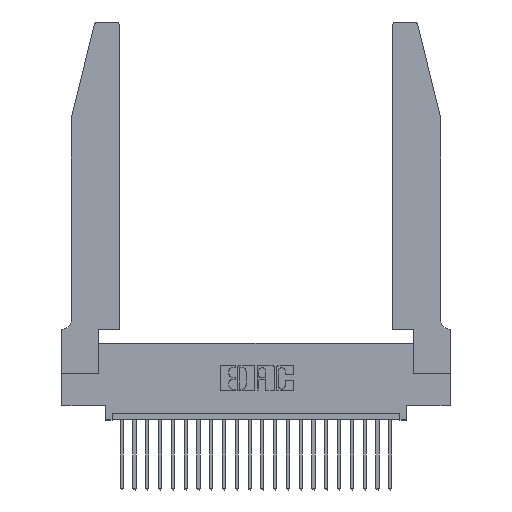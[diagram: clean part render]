
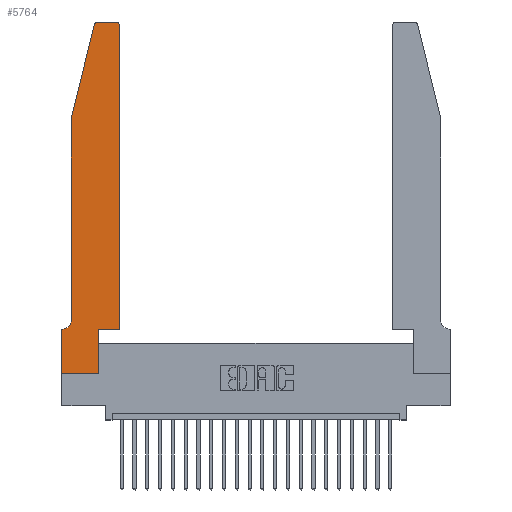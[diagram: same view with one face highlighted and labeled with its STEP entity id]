
A CAD part, top view. The second image highlights one B-rep face of the part: STEP entity #5764.
In plain terms, the highlighted planar face has unit normal (0, 0, 1).
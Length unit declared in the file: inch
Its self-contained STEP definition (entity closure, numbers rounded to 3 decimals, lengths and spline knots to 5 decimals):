
#12 = DIRECTION ( 'NONE',  ( 0., 0., 1. ) ) ;
#119 = EDGE_CURVE ( 'NONE', #18789, #23798, #5246, .T. ) ;
#302 = VECTOR ( 'NONE', #23434, 39.37008 ) ;
#432 = EDGE_CURVE ( 'NONE', #23798, #5064, #21632, .T. ) ;
#566 = VERTEX_POINT ( 'NONE', #6598 ) ;
#702 = EDGE_CURVE ( 'NONE', #5064, #22696, #14632, .T. ) ;
#795 = ORIENTED_EDGE ( 'NONE', *, *, #19122, .T. ) ;
#945 = VERTEX_POINT ( 'NONE', #11610 ) ;
#1464 = CARTESIAN_POINT ( 'NONE',  ( 0.0755, 2., 0.37 ) ) ;
#1549 = DIRECTION ( 'NONE',  ( 1., 0., 0. ) ) ;
#2223 = DIRECTION ( 'NONE',  ( 1., 0., 0. ) ) ;
#2553 = CARTESIAN_POINT ( 'NONE',  ( 0.0755, 0.42, 0.37 ) ) ;
#2623 = ORIENTED_EDGE ( 'NONE', *, *, #15102, .T. ) ;
#2695 = VECTOR ( 'NONE', #16484, 39.37008 ) ;
#2698 = ORIENTED_EDGE ( 'NONE', *, *, #7828, .T. ) ;
#2810 = DIRECTION ( 'NONE',  ( 1., 0., 0. ) ) ;
#2921 = VECTOR ( 'NONE', #13179, 39.37008 ) ;
#3017 = CARTESIAN_POINT ( 'NONE',  ( 0.0755, 2., 0.37 ) ) ;
#3178 = VECTOR ( 'NONE', #5280, 39.37008 ) ;
#3492 = ORIENTED_EDGE ( 'NONE', *, *, #9373, .T. ) ;
#4136 = DIRECTION ( 'NONE',  ( 0., 1., 0. ) ) ;
#4333 = CIRCLE ( 'NONE', #5457, 0.03 ) ;
#4637 = VERTEX_POINT ( 'NONE', #20187 ) ;
#4794 = CARTESIAN_POINT ( 'NONE',  ( 0., 0.35, 0.37 ) ) ;
#4965 = CARTESIAN_POINT ( 'NONE',  ( 0., 0., 0.37 ) ) ;
#5064 = VERTEX_POINT ( 'NONE', #14235 ) ;
#5246 = LINE ( 'NONE', #9996, #302 ) ;
#5280 = DIRECTION ( 'NONE',  ( -0.239, -0.971, 0. ) ) ;
#5457 = AXIS2_PLACEMENT_3D ( 'NONE', #12424, #21608, #2810 ) ;
#5468 = CARTESIAN_POINT ( 'NONE',  ( 0.2605, 2.75, 0.37 ) ) ;
#5632 = EDGE_CURVE ( 'NONE', #21778, #21929, #9237, .T. ) ;
#5662 = VECTOR ( 'NONE', #16864, 39.37008 ) ;
#5764 = ADVANCED_FACE ( 'NONE', ( #15664 ), #17740, .T. ) ;
#6284 = CARTESIAN_POINT ( 'NONE',  ( 0.2865, 0.35, 0.37 ) ) ;
#6301 = AXIS2_PLACEMENT_3D ( 'NONE', #13717, #21052, #11763 ) ;
#6598 = CARTESIAN_POINT ( 'NONE',  ( 0.4505, 2.72, 0.37 ) ) ;
#6871 = EDGE_LOOP ( 'NONE', ( #10457, #3492, #2623, #7031, #16558, #19944, #7434, #2698, #12664, #17879, #9995, #795 ) ) ;
#7031 = ORIENTED_EDGE ( 'NONE', *, *, #119, .T. ) ;
#7434 = ORIENTED_EDGE ( 'NONE', *, *, #8720, .T. ) ;
#7692 = LINE ( 'NONE', #4965, #2695 ) ;
#7712 = DIRECTION ( 'NONE',  ( 0., 1., 0. ) ) ;
#7788 = CARTESIAN_POINT ( 'NONE',  ( 0.4505, 0.35, 0.37 ) ) ;
#7828 = EDGE_CURVE ( 'NONE', #945, #21778, #7692, .T. ) ;
#7903 = LINE ( 'NONE', #1464, #3178 ) ;
#8044 = VECTOR ( 'NONE', #4136, 39.37008 ) ;
#8320 = CARTESIAN_POINT ( 'NONE',  ( 0.25487, 2.72718, 0.37 ) ) ;
#8557 = AXIS2_PLACEMENT_3D ( 'NONE', #10317, #10395, #1549 ) ;
#8720 = EDGE_CURVE ( 'NONE', #22696, #945, #19917, .T. ) ;
#8729 = DIRECTION ( 'NONE',  ( -1., 0., 0. ) ) ;
#9237 = LINE ( 'NONE', #6284, #8044 ) ;
#9296 = CARTESIAN_POINT ( 'NONE',  ( 0.2865, 0., 0.37 ) ) ;
#9363 = LINE ( 'NONE', #7788, #18984 ) ;
#9373 = EDGE_CURVE ( 'NONE', #21474, #12568, #4333, .T. ) ;
#9563 = CARTESIAN_POINT ( 'NONE',  ( 0., 0., 0.37 ) ) ;
#9755 = CARTESIAN_POINT ( 'NONE',  ( 0.4505, 0.35, 0.37 ) ) ;
#9862 = AXIS2_PLACEMENT_3D ( 'NONE', #20445, #12, #16941 ) ;
#9995 = ORIENTED_EDGE ( 'NONE', *, *, #19841, .T. ) ;
#9996 = CARTESIAN_POINT ( 'NONE',  ( 0.0755, 2., 0.37 ) ) ;
#10317 = CARTESIAN_POINT ( 'NONE',  ( 0., 0.35, 0.37 ) ) ;
#10395 = DIRECTION ( 'NONE',  ( 0., 0., 1. ) ) ;
#10457 = ORIENTED_EDGE ( 'NONE', *, *, #12862, .T. ) ;
#11610 = CARTESIAN_POINT ( 'NONE',  ( 0., 0., 0.37 ) ) ;
#11763 = DIRECTION ( 'NONE',  ( -1., 0., 0. ) ) ;
#12424 = CARTESIAN_POINT ( 'NONE',  ( 0.284, 2.72, 0.37 ) ) ;
#12568 = VERTEX_POINT ( 'NONE', #8320 ) ;
#12664 = ORIENTED_EDGE ( 'NONE', *, *, #5632, .T. ) ;
#12862 = EDGE_CURVE ( 'NONE', #4637, #21474, #13573, .T. ) ;
#13179 = DIRECTION ( 'NONE',  ( 0., -1., 0. ) ) ;
#13573 = LINE ( 'NONE', #5468, #5662 ) ;
#13717 = CARTESIAN_POINT ( 'NONE',  ( 0.0055, 0.42, 0.37 ) ) ;
#13953 = VECTOR ( 'NONE', #2223, 39.37008 ) ;
#14235 = CARTESIAN_POINT ( 'NONE',  ( 0.0055, 0.35, 0.37 ) ) ;
#14632 = LINE ( 'NONE', #23488, #21041 ) ;
#15102 = EDGE_CURVE ( 'NONE', #12568, #18789, #7903, .T. ) ;
#15664 = FACE_OUTER_BOUND ( 'NONE', #6871, .T. ) ;
#16484 = DIRECTION ( 'NONE',  ( 1., 0., 0. ) ) ;
#16558 = ORIENTED_EDGE ( 'NONE', *, *, #432, .T. ) ;
#16864 = DIRECTION ( 'NONE',  ( -1., 0., 0. ) ) ;
#16941 = DIRECTION ( 'NONE',  ( 1., 0., 0. ) ) ;
#17706 = LINE ( 'NONE', #9755, #13953 ) ;
#17740 = PLANE ( 'NONE',  #8557 ) ;
#17879 = ORIENTED_EDGE ( 'NONE', *, *, #22461, .T. ) ;
#18166 = VERTEX_POINT ( 'NONE', #21372 ) ;
#18789 = VERTEX_POINT ( 'NONE', #3017 ) ;
#18936 = CARTESIAN_POINT ( 'NONE',  ( 0.2865, 0.35, 0.37 ) ) ;
#18984 = VECTOR ( 'NONE', #7712, 39.37008 ) ;
#19122 = EDGE_CURVE ( 'NONE', #566, #4637, #23384, .T. ) ;
#19672 = CARTESIAN_POINT ( 'NONE',  ( 0.284, 2.75, 0.37 ) ) ;
#19841 = EDGE_CURVE ( 'NONE', #18166, #566, #9363, .T. ) ;
#19917 = LINE ( 'NONE', #9563, #2921 ) ;
#19944 = ORIENTED_EDGE ( 'NONE', *, *, #702, .T. ) ;
#20187 = CARTESIAN_POINT ( 'NONE',  ( 0.4205, 2.75, 0.37 ) ) ;
#20445 = CARTESIAN_POINT ( 'NONE',  ( 0.4205, 2.72, 0.37 ) ) ;
#21041 = VECTOR ( 'NONE', #8729, 39.37008 ) ;
#21052 = DIRECTION ( 'NONE',  ( 0., 0., -1. ) ) ;
#21372 = CARTESIAN_POINT ( 'NONE',  ( 0.4505, 0.35, 0.37 ) ) ;
#21474 = VERTEX_POINT ( 'NONE', #19672 ) ;
#21608 = DIRECTION ( 'NONE',  ( 0., 0., 1. ) ) ;
#21632 = CIRCLE ( 'NONE', #6301, 0.07 ) ;
#21778 = VERTEX_POINT ( 'NONE', #9296 ) ;
#21929 = VERTEX_POINT ( 'NONE', #18936 ) ;
#22461 = EDGE_CURVE ( 'NONE', #21929, #18166, #17706, .T. ) ;
#22696 = VERTEX_POINT ( 'NONE', #4794 ) ;
#23384 = CIRCLE ( 'NONE', #9862, 0.03 ) ;
#23434 = DIRECTION ( 'NONE',  ( 0., -1., 0. ) ) ;
#23488 = CARTESIAN_POINT ( 'NONE',  ( 0.0755, 0.35, 0.37 ) ) ;
#23798 = VERTEX_POINT ( 'NONE', #2553 ) ;
